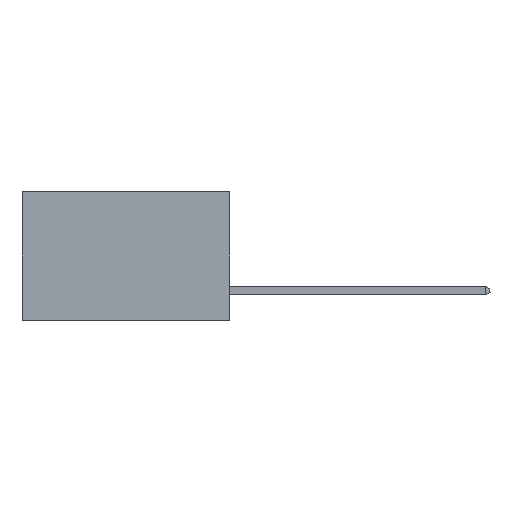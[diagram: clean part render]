
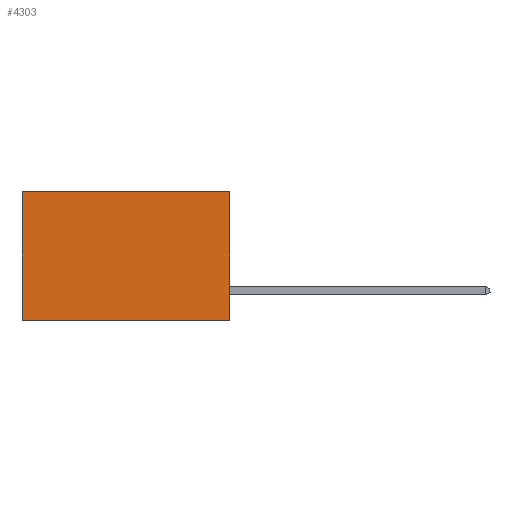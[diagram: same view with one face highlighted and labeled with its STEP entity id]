
A CAD part, left-side view. The second image highlights one B-rep face of the part: STEP entity #4303.
In plain terms, the highlighted planar face has unit normal (-1, 0, 0).
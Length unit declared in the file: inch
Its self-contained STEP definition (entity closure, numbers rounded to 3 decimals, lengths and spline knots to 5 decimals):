
#456 = CARTESIAN_POINT ( 'NONE',  ( 0.298, 0., 0. ) ) ;
#506 = FACE_OUTER_BOUND ( 'NONE', #2670, .T. ) ;
#541 = ORIENTED_EDGE ( 'NONE', *, *, #2085, .T. ) ;
#548 = CARTESIAN_POINT ( 'NONE',  ( 0.298, 0.6, -0.37 ) ) ;
#963 = CARTESIAN_POINT ( 'NONE',  ( 0.298, 0.6, 0. ) ) ;
#1212 = VECTOR ( 'NONE', #2851, 39.37008 ) ;
#1633 = VERTEX_POINT ( 'NONE', #548 ) ;
#1660 = VERTEX_POINT ( 'NONE', #456 ) ;
#1925 = CARTESIAN_POINT ( 'NONE',  ( 0.298, 0., -0.37 ) ) ;
#2021 = LINE ( 'NONE', #3006, #6078 ) ;
#2034 = EDGE_CURVE ( 'NONE', #1660, #7287, #3288, .T. ) ;
#2085 = EDGE_CURVE ( 'NONE', #6906, #1633, #4558, .T. ) ;
#2670 = EDGE_LOOP ( 'NONE', ( #541, #6347, #7027, #5763 ) ) ;
#2700 = DIRECTION ( 'NONE',  ( 1., 0., 0. ) ) ;
#2851 = DIRECTION ( 'NONE',  ( 0., 1., 0. ) ) ;
#3006 = CARTESIAN_POINT ( 'NONE',  ( 0.298, 0., 0. ) ) ;
#3111 = EDGE_CURVE ( 'NONE', #7287, #1633, #3504, .T. ) ;
#3288 = LINE ( 'NONE', #8259, #6761 ) ;
#3472 = PLANE ( 'NONE',  #5802 ) ;
#3504 = LINE ( 'NONE', #5368, #1212 ) ;
#4116 = VECTOR ( 'NONE', #6210, 39.37008 ) ;
#4303 = ADVANCED_FACE ( 'NONE', ( #506 ), #3472, .F. ) ;
#4310 = EDGE_CURVE ( 'NONE', #1660, #6906, #2021, .T. ) ;
#4558 = LINE ( 'NONE', #4877, #4116 ) ;
#4877 = CARTESIAN_POINT ( 'NONE',  ( 0.298, 0.6, 0. ) ) ;
#5368 = CARTESIAN_POINT ( 'NONE',  ( 0.298, 0., -0.37 ) ) ;
#5602 = CARTESIAN_POINT ( 'NONE',  ( 0.298, 0., 0. ) ) ;
#5763 = ORIENTED_EDGE ( 'NONE', *, *, #4310, .T. ) ;
#5802 = AXIS2_PLACEMENT_3D ( 'NONE', #5602, #2700, #6891 ) ;
#6078 = VECTOR ( 'NONE', #6939, 39.37008 ) ;
#6210 = DIRECTION ( 'NONE',  ( 0., 0., -1. ) ) ;
#6347 = ORIENTED_EDGE ( 'NONE', *, *, #3111, .F. ) ;
#6761 = VECTOR ( 'NONE', #8495, 39.37008 ) ;
#6891 = DIRECTION ( 'NONE',  ( 0., 0., -1. ) ) ;
#6906 = VERTEX_POINT ( 'NONE', #963 ) ;
#6939 = DIRECTION ( 'NONE',  ( 0., 1., 0. ) ) ;
#7027 = ORIENTED_EDGE ( 'NONE', *, *, #2034, .F. ) ;
#7287 = VERTEX_POINT ( 'NONE', #1925 ) ;
#8259 = CARTESIAN_POINT ( 'NONE',  ( 0.298, 0., 0. ) ) ;
#8495 = DIRECTION ( 'NONE',  ( 0., 0., -1. ) ) ;
